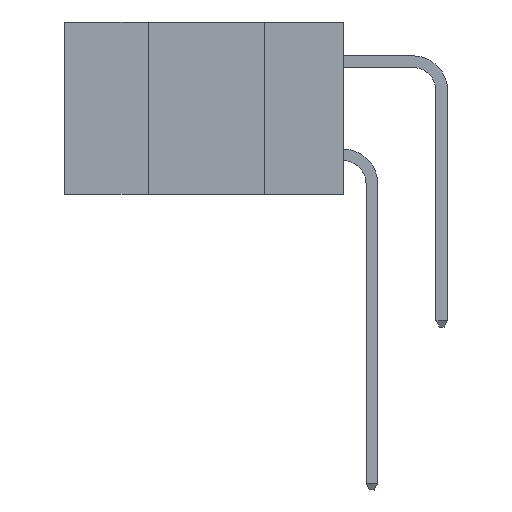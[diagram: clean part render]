
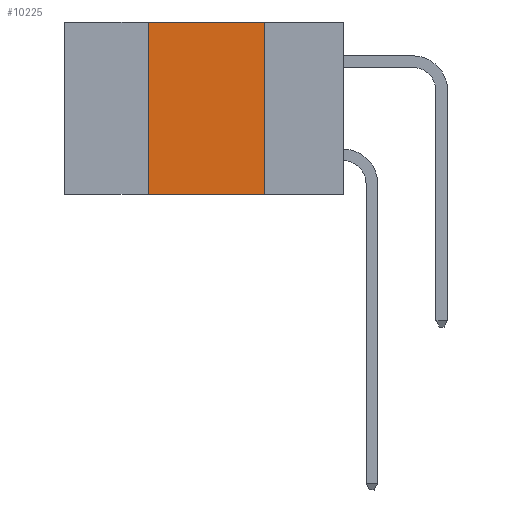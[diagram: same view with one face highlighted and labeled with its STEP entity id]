
A CAD part, left-side view. The second image highlights one B-rep face of the part: STEP entity #10225.
In plain terms, the highlighted planar face has unit normal (-1, 0, 0).
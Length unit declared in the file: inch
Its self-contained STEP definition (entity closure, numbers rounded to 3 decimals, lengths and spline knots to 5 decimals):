
#299 = EDGE_CURVE ( 'NONE', #14234, #4457, #8384, .T. ) ;
#1659 = CARTESIAN_POINT ( 'NONE',  ( 0., 0.6, 0. ) ) ;
#2437 = DIRECTION ( 'NONE',  ( 1., 0., 0. ) ) ;
#3041 = CARTESIAN_POINT ( 'NONE',  ( 0., 0.17, 0. ) ) ;
#3319 = CARTESIAN_POINT ( 'NONE',  ( 0., 0.6, -0.37 ) ) ;
#3738 = CARTESIAN_POINT ( 'NONE',  ( 0., 0.42, -0.37 ) ) ;
#3775 = FACE_OUTER_BOUND ( 'NONE', #14926, .T. ) ;
#3825 = CARTESIAN_POINT ( 'NONE',  ( 0., 0.42, 0. ) ) ;
#4223 = CARTESIAN_POINT ( 'NONE',  ( 0., 0.17, -0.37 ) ) ;
#4457 = VERTEX_POINT ( 'NONE', #9162 ) ;
#4731 = ORIENTED_EDGE ( 'NONE', *, *, #9078, .T. ) ;
#5058 = VECTOR ( 'NONE', #9021, 39.37008 ) ;
#5397 = VECTOR ( 'NONE', #13481, 39.37008 ) ;
#5916 = DIRECTION ( 'NONE',  ( 0., -1., 0. ) ) ;
#6315 = EDGE_CURVE ( 'NONE', #4457, #6324, #11421, .T. ) ;
#6324 = VERTEX_POINT ( 'NONE', #4223 ) ;
#7205 = PLANE ( 'NONE',  #13402 ) ;
#7635 = VECTOR ( 'NONE', #11662, 39.37008 ) ;
#8002 = VECTOR ( 'NONE', #5916, 39.37008 ) ;
#8384 = LINE ( 'NONE', #1659, #8002 ) ;
#9021 = DIRECTION ( 'NONE',  ( 0., 0., -1. ) ) ;
#9078 = EDGE_CURVE ( 'NONE', #9981, #6324, #10061, .T. ) ;
#9162 = CARTESIAN_POINT ( 'NONE',  ( 0., 0.17, 0. ) ) ;
#9981 = VERTEX_POINT ( 'NONE', #3738 ) ;
#10061 = LINE ( 'NONE', #3319, #7635 ) ;
#10225 = ADVANCED_FACE ( 'NONE', ( #3775 ), #7205, .F. ) ;
#10748 = CARTESIAN_POINT ( 'NONE',  ( 0., 0.6, 0. ) ) ;
#10795 = DIRECTION ( 'NONE',  ( 0., 0., -1. ) ) ;
#11421 = LINE ( 'NONE', #3041, #5058 ) ;
#11463 = CARTESIAN_POINT ( 'NONE',  ( 0., 0.42, 0. ) ) ;
#11662 = DIRECTION ( 'NONE',  ( 0., -1., 0. ) ) ;
#11718 = ORIENTED_EDGE ( 'NONE', *, *, #6315, .F. ) ;
#11771 = LINE ( 'NONE', #3825, #5397 ) ;
#12721 = ORIENTED_EDGE ( 'NONE', *, *, #299, .F. ) ;
#12814 = EDGE_CURVE ( 'NONE', #9981, #14234, #11771, .T. ) ;
#13402 = AXIS2_PLACEMENT_3D ( 'NONE', #10748, #2437, #10795 ) ;
#13481 = DIRECTION ( 'NONE',  ( 0., 0., 1. ) ) ;
#14012 = ORIENTED_EDGE ( 'NONE', *, *, #12814, .F. ) ;
#14234 = VERTEX_POINT ( 'NONE', #11463 ) ;
#14926 = EDGE_LOOP ( 'NONE', ( #11718, #12721, #14012, #4731 ) ) ;
